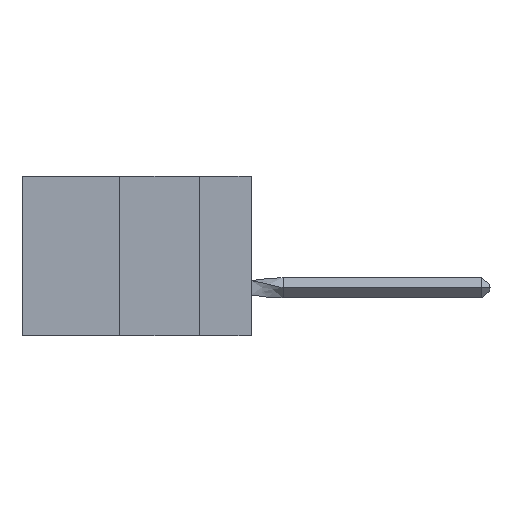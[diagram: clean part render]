
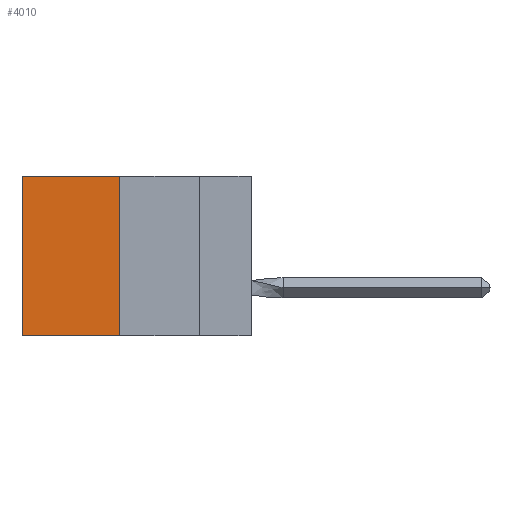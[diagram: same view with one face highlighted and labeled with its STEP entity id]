
A CAD part, left-side view. The second image highlights one B-rep face of the part: STEP entity #4010.
In plain terms, the highlighted planar face has unit normal (-1, 0, 0).
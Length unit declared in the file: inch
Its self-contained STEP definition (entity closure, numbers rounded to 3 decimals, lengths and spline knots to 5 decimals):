
#804 = PLANE ( 'NONE',  #6874 ) ;
#807 = FACE_OUTER_BOUND ( 'NONE', #1962, .T. ) ;
#1097 = EDGE_CURVE ( 'NONE', #16059, #6303, #18684, .T. ) ;
#1385 = VECTOR ( 'NONE', #8567, 39.37008 ) ;
#1962 = EDGE_LOOP ( 'NONE', ( #14744, #4847, #17196, #3263 ) ) ;
#2470 = DIRECTION ( 'NONE',  ( 0., 0., -1. ) ) ;
#2608 = LINE ( 'NONE', #5193, #18283 ) ;
#3263 = ORIENTED_EDGE ( 'NONE', *, *, #7820, .T. ) ;
#4010 = ADVANCED_FACE ( 'NONE', ( #807 ), #804, .F. ) ;
#4847 = ORIENTED_EDGE ( 'NONE', *, *, #1097, .F. ) ;
#5193 = CARTESIAN_POINT ( 'NONE',  ( 0.305, 0.413, -0.5 ) ) ;
#5214 = CARTESIAN_POINT ( 'NONE',  ( 0.305, 0.72, -0.5 ) ) ;
#5652 = VECTOR ( 'NONE', #18437, 39.37008 ) ;
#5886 = LINE ( 'NONE', #5214, #5652 ) ;
#5892 = VERTEX_POINT ( 'NONE', #8694 ) ;
#6303 = VERTEX_POINT ( 'NONE', #15780 ) ;
#6839 = EDGE_CURVE ( 'NONE', #11798, #6303, #5886, .T. ) ;
#6874 = AXIS2_PLACEMENT_3D ( 'NONE', #7124, #8516, #17214 ) ;
#7124 = CARTESIAN_POINT ( 'NONE',  ( 0.305, 0.413, -0.5 ) ) ;
#7543 = LINE ( 'NONE', #18727, #1385 ) ;
#7820 = EDGE_CURVE ( 'NONE', #5892, #11798, #7543, .T. ) ;
#7917 = DIRECTION ( 'NONE',  ( 0., 1., 0. ) ) ;
#8516 = DIRECTION ( 'NONE',  ( 1., 0., 0. ) ) ;
#8550 = EDGE_CURVE ( 'NONE', #5892, #16059, #2608, .T. ) ;
#8567 = DIRECTION ( 'NONE',  ( 0., 1., 0. ) ) ;
#8694 = CARTESIAN_POINT ( 'NONE',  ( 0.305, 0.413, 0. ) ) ;
#9188 = CARTESIAN_POINT ( 'NONE',  ( 0.305, 0.413, -0.5 ) ) ;
#9483 = CARTESIAN_POINT ( 'NONE',  ( 0.305, 0.72, 0. ) ) ;
#9577 = CARTESIAN_POINT ( 'NONE',  ( 0.305, 0.413, -0.5 ) ) ;
#9592 = VECTOR ( 'NONE', #7917, 39.37008 ) ;
#11798 = VERTEX_POINT ( 'NONE', #9483 ) ;
#14744 = ORIENTED_EDGE ( 'NONE', *, *, #6839, .T. ) ;
#15780 = CARTESIAN_POINT ( 'NONE',  ( 0.305, 0.72, -0.5 ) ) ;
#16059 = VERTEX_POINT ( 'NONE', #9577 ) ;
#17196 = ORIENTED_EDGE ( 'NONE', *, *, #8550, .F. ) ;
#17214 = DIRECTION ( 'NONE',  ( 0., 0., -1. ) ) ;
#18283 = VECTOR ( 'NONE', #2470, 39.37008 ) ;
#18437 = DIRECTION ( 'NONE',  ( 0., 0., -1. ) ) ;
#18684 = LINE ( 'NONE', #9188, #9592 ) ;
#18727 = CARTESIAN_POINT ( 'NONE',  ( 0.305, 0.413, 0. ) ) ;
